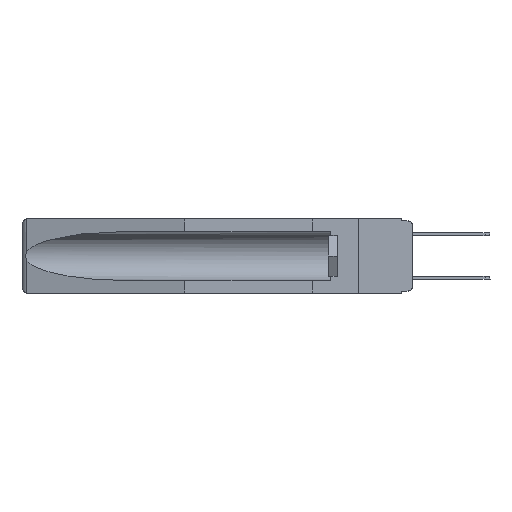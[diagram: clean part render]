
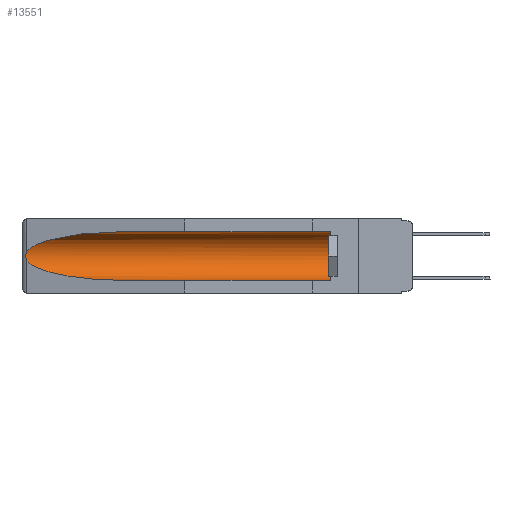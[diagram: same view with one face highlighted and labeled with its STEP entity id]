
A CAD part, left-side view. The second image highlights one B-rep face of the part: STEP entity #13551.
In plain terms, the highlighted cylindrical face has radius 2.857 mm (diameter 5.715 mm), a partial arc.
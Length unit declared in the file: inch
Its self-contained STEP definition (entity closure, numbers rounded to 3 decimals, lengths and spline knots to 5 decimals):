
#476 = AXIS2_PLACEMENT_3D ( 'NONE', #18392, #13161, #17987 ) ;
#590 = VERTEX_POINT ( 'NONE', #16858 ) ;
#820 = CARTESIAN_POINT ( 'NONE',  ( 0.21114, 1.30732, -0.059 ) ) ;
#1416 = EDGE_LOOP ( 'NONE', ( #13203, #13804, #12242, #10307, #17152, #14527 ) ) ;
#1494 = CARTESIAN_POINT ( 'NONE',  ( 0.155, 0.126, -0.059 ) ) ;
#1772 = CARTESIAN_POINT ( 'NONE',  ( 0.26537, 1.52718, -0.19328 ) ) ;
#1910 = CARTESIAN_POINT ( 'NONE',  ( 0.21114, 1.30732, -0.284 ) ) ;
#1976 = CARTESIAN_POINT ( 'NONE',  ( 0.26597, 1.52961, -0.15275 ) ) ;
#1983 = CARTESIAN_POINT ( 'NONE',  ( 0.26537, 1.52718, -0.14972 ) ) ;
#2142 = CARTESIAN_POINT ( 'NONE',  ( 0.155, 1.07973, -0.059 ) ) ;
#4135 = VERTEX_POINT ( 'NONE', #1494 ) ;
#4795 = LINE ( 'NONE', #14264, #16912 ) ;
#5763 = VERTEX_POINT ( 'NONE', #5982 ) ;
#5960 = CIRCLE ( 'NONE', #476, 0.1125 ) ;
#5982 = CARTESIAN_POINT ( 'NONE',  ( 0.155, 1.07973, -0.059 ) ) ;
#6362 = CARTESIAN_POINT ( 'NONE',  ( 0.155, -0.30754, -0.1715 ) ) ;
#6455 = DIRECTION ( 'NONE',  ( 0., 1., 0. ) ) ;
#6580 = CARTESIAN_POINT ( 'NONE',  ( 0.2675, 1.53308, -0.17534 ) ) ;
#7177 = DIRECTION ( 'NONE',  ( 0., 1., 0. ) ) ;
#8089 = CARTESIAN_POINT ( 'NONE',  ( 0.2673, 1.53269, -0.17917 ) ) ;
#8257 = CYLINDRICAL_SURFACE ( 'NONE', #12076, 0.1125 ) ;
#8266 = CARTESIAN_POINT ( 'NONE',  ( 0.25451, 1.48313, -0.09465 ) ) ;
#8279 = EDGE_CURVE ( 'NONE', #4135, #5763, #14481, .T. ) ;
#8369 = CARTESIAN_POINT ( 'NONE',  ( 0.26537, 1.52718, -0.14972 ) ) ;
#8783 = VECTOR ( 'NONE', #7177, 39.37008 ) ;
#9218 =( BOUNDED_CURVE ( )  B_SPLINE_CURVE ( 3, ( #2142, #820, #8266, #8369 ),
 .UNSPECIFIED., .F., .T. ) 
 B_SPLINE_CURVE_WITH_KNOTS ( ( 4, 4 ),
 ( 4.71239, 6.08839 ),
 .UNSPECIFIED. ) 
 CURVE ( )  GEOMETRIC_REPRESENTATION_ITEM ( )  RATIONAL_B_SPLINE_CURVE ( ( 1., 0.848, 0.848, 1. ) ) 
 REPRESENTATION_ITEM ( '' )  );
#9251 = EDGE_CURVE ( 'NONE', #12749, #18141, #12830, .T. ) ;
#9621 = CARTESIAN_POINT ( 'NONE',  ( 0.26654, 1.53092, -0.15636 ) ) ;
#9752 = CARTESIAN_POINT ( 'NONE',  ( 0.155, 1.07973, -0.284 ) ) ;
#10307 = ORIENTED_EDGE ( 'NONE', *, *, #16209, .F. ) ;
#10959 = DIRECTION ( 'NONE',  ( 0., 1., 0. ) ) ;
#11142 = VERTEX_POINT ( 'NONE', #1983 ) ;
#12019 = CARTESIAN_POINT ( 'NONE',  ( 0.155, 1.07973, -0.284 ) ) ;
#12076 = AXIS2_PLACEMENT_3D ( 'NONE', #6362, #6455, #14425 ) ;
#12242 = ORIENTED_EDGE ( 'NONE', *, *, #9251, .T. ) ;
#12360 = CARTESIAN_POINT ( 'NONE',  ( 0.26597, 1.5296, -0.19026 ) ) ;
#12462 = CARTESIAN_POINT ( 'NONE',  ( 0.2673, 1.5327, -0.16383 ) ) ;
#12749 = VERTEX_POINT ( 'NONE', #19856 ) ;
#12830 =( BOUNDED_CURVE ( )  B_SPLINE_CURVE ( 3, ( #14482, #12897, #1910, #9752 ),
 .UNSPECIFIED., .F., .T. ) 
 B_SPLINE_CURVE_WITH_KNOTS ( ( 4, 4 ),
 ( 0.1948, 1.5708 ),
 .UNSPECIFIED. ) 
 CURVE ( )  GEOMETRIC_REPRESENTATION_ITEM ( )  RATIONAL_B_SPLINE_CURVE ( ( 1., 0.848, 0.848, 1. ) ) 
 REPRESENTATION_ITEM ( '' )  );
#12897 = CARTESIAN_POINT ( 'NONE',  ( 0.25451, 1.48313, -0.24835 ) ) ;
#13161 = DIRECTION ( 'NONE',  ( 0., -1., 0. ) ) ;
#13203 = ORIENTED_EDGE ( 'NONE', *, *, #16772, .T. ) ;
#13551 = ADVANCED_FACE ( 'NONE', ( #16646 ), #8257, .F. ) ;
#13804 = ORIENTED_EDGE ( 'NONE', *, *, #17511, .T. ) ;
#14117 = B_SPLINE_CURVE_WITH_KNOTS ( 'NONE', 3,
 ( #18472, #1976, #9621, #12462, #15777, #6580, #8089, #14266, #12360, #1772 ),
 .UNSPECIFIED., .F., .F.,
 ( 4, 2, 2, 2, 4 ),
 ( 0., 0.00029, 0.00058, 0.00087, 0.00117 ),
 .UNSPECIFIED. ) ;
#14254 = EDGE_CURVE ( 'NONE', #590, #4135, #5960, .T. ) ;
#14264 = CARTESIAN_POINT ( 'NONE',  ( 0.155, -0.30754, -0.284 ) ) ;
#14266 = CARTESIAN_POINT ( 'NONE',  ( 0.26655, 1.53094, -0.18657 ) ) ;
#14425 = DIRECTION ( 'NONE',  ( 0., 0., 1. ) ) ;
#14481 = LINE ( 'NONE', #17877, #8783 ) ;
#14482 = CARTESIAN_POINT ( 'NONE',  ( 0.26537, 1.52718, -0.19328 ) ) ;
#14527 = ORIENTED_EDGE ( 'NONE', *, *, #8279, .T. ) ;
#15777 = CARTESIAN_POINT ( 'NONE',  ( 0.2675, 1.53308, -0.16763 ) ) ;
#16209 = EDGE_CURVE ( 'NONE', #590, #18141, #4795, .T. ) ;
#16646 = FACE_OUTER_BOUND ( 'NONE', #1416, .T. ) ;
#16772 = EDGE_CURVE ( 'NONE', #5763, #11142, #9218, .T. ) ;
#16858 = CARTESIAN_POINT ( 'NONE',  ( 0.155, 0.126, -0.284 ) ) ;
#16912 = VECTOR ( 'NONE', #10959, 39.37008 ) ;
#17152 = ORIENTED_EDGE ( 'NONE', *, *, #14254, .T. ) ;
#17511 = EDGE_CURVE ( 'NONE', #11142, #12749, #14117, .T. ) ;
#17877 = CARTESIAN_POINT ( 'NONE',  ( 0.155, -0.30754, -0.059 ) ) ;
#17987 = DIRECTION ( 'NONE',  ( 0., 0., 1. ) ) ;
#18141 = VERTEX_POINT ( 'NONE', #12019 ) ;
#18392 = CARTESIAN_POINT ( 'NONE',  ( 0.155, 0.126, -0.1715 ) ) ;
#18472 = CARTESIAN_POINT ( 'NONE',  ( 0.26537, 1.52718, -0.14972 ) ) ;
#19856 = CARTESIAN_POINT ( 'NONE',  ( 0.26537, 1.52718, -0.19328 ) ) ;
